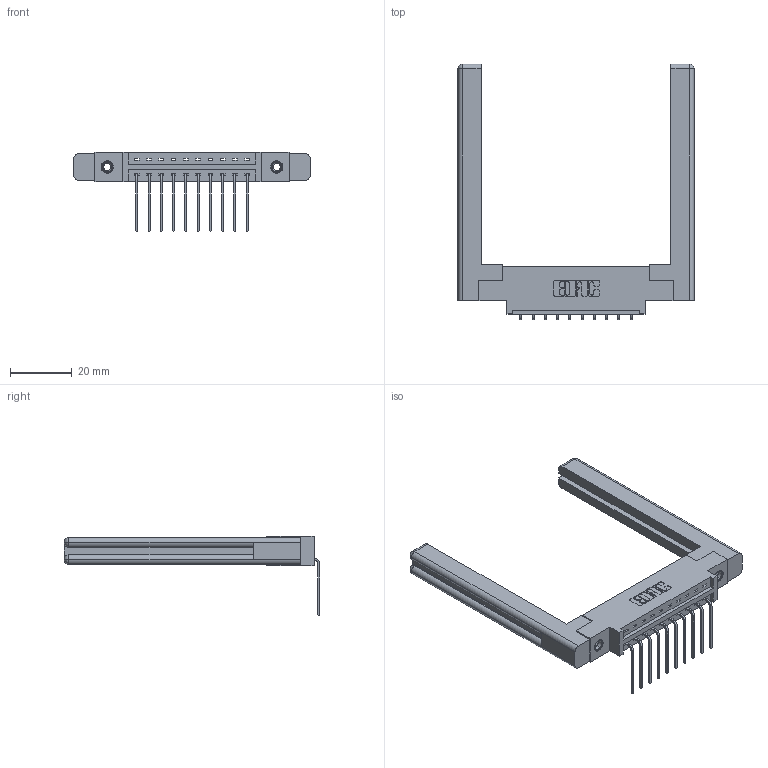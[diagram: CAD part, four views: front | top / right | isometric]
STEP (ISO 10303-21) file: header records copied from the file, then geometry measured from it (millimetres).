
FILE_DESCRIPTION (( 'STEP AP203' ), '1' );
FILE_NAME ('387-010-559-658.STEP', '2019-10-02T11:48:45', ( '' ), ( '' ), 'SwSTEP 2.0', 'SolidWorks 2016', '' );
FILE_SCHEMA (( 'CONFIG_CONTROL_DESIGN' ));
Length unit declared in the file: inch
Products named in the file (5): 307-220-058; 345-292-001_558 559 Tail - 1; 387-010-559-658; 337 Part_0.170 Offset - 0.156 Dia-TI; 345-250-001_345-250-001-102
Assembly tree (15 placements, depth 2):
  387-010-559-658
    337 Part_0.170 Offset - 0.156 Dia-TI
    345-292-001_558 559 Tail - 1  x10
    345-250-001_345-250-001-102  x2
    307-220-058  x2
Bounding box: 76.25 x 82.49 x 25.53 mm (x, y, z)
Volume: 14602.5 mm3; surface area: 13025 mm2
Topology: 15 solids, 15 shells, 900 faces, 2617 edges, 1718 vertices
Faces by surface type: plane 638, cylinder 238, cone 12, torus 12
Entity records: 14422 total; most frequent: CARTESIAN_POINT 2511, ORIENTED_EDGE 2396, DIRECTION 2198, EDGE_CURVE 1198, LINE 1022, VECTOR 1022, VERTEX_POINT 790, AXIS2_PLACEMENT_3D 588
